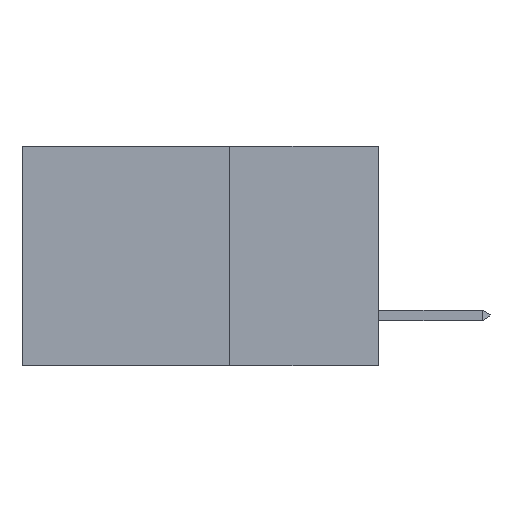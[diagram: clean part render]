
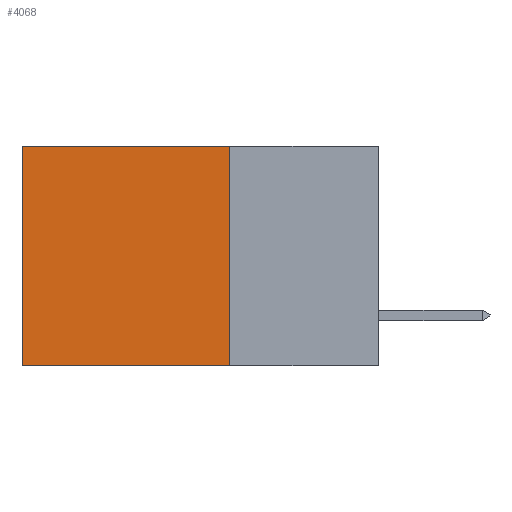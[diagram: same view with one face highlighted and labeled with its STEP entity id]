
A CAD part, left-side view. The second image highlights one B-rep face of the part: STEP entity #4068.
In plain terms, the highlighted planar face has unit normal (-1, 0, 0).
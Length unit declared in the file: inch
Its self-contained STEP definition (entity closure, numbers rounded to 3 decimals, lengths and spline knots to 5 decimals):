
#533 = DIRECTION ( 'NONE',  ( 0., 0., -1. ) ) ;
#1147 = LINE ( 'NONE', #7698, #16302 ) ;
#1148 = DIRECTION ( 'NONE',  ( 0., 0., -1. ) ) ;
#1410 = CARTESIAN_POINT ( 'NONE',  ( 0.2615, 0.25, -0.37 ) ) ;
#2628 = EDGE_LOOP ( 'NONE', ( #19874, #8429, #19953, #14181 ) ) ;
#3042 = EDGE_CURVE ( 'NONE', #7414, #20950, #13344, .T. ) ;
#4068 = ADVANCED_FACE ( 'NONE', ( #11348 ), #14703, .F. ) ;
#4478 = DIRECTION ( 'NONE',  ( 1., 0., 0. ) ) ;
#6348 = CARTESIAN_POINT ( 'NONE',  ( 0.2615, 0.25, -0.37 ) ) ;
#7414 = VERTEX_POINT ( 'NONE', #17728 ) ;
#7698 = CARTESIAN_POINT ( 'NONE',  ( 0.2615, 0.25, -0.37 ) ) ;
#7756 = VECTOR ( 'NONE', #13447, 39.37008 ) ;
#8429 = ORIENTED_EDGE ( 'NONE', *, *, #12754, .F. ) ;
#8626 = CARTESIAN_POINT ( 'NONE',  ( 0.2615, 0.6, -0.37 ) ) ;
#8818 = CARTESIAN_POINT ( 'NONE',  ( 0.2615, 0.6, 0. ) ) ;
#8958 = CARTESIAN_POINT ( 'NONE',  ( 0.2615, 0.25, -0.37 ) ) ;
#9487 = VECTOR ( 'NONE', #533, 39.37008 ) ;
#10352 = AXIS2_PLACEMENT_3D ( 'NONE', #6348, #4478, #1148 ) ;
#10924 = EDGE_CURVE ( 'NONE', #20950, #11629, #19082, .T. ) ;
#10967 = EDGE_CURVE ( 'NONE', #7414, #18882, #17422, .T. ) ;
#11257 = VECTOR ( 'NONE', #19298, 39.37008 ) ;
#11348 = FACE_OUTER_BOUND ( 'NONE', #2628, .T. ) ;
#11629 = VERTEX_POINT ( 'NONE', #21600 ) ;
#12754 = EDGE_CURVE ( 'NONE', #18882, #11629, #1147, .T. ) ;
#13344 = LINE ( 'NONE', #18709, #7756 ) ;
#13447 = DIRECTION ( 'NONE',  ( 0., 1., 0. ) ) ;
#14181 = ORIENTED_EDGE ( 'NONE', *, *, #3042, .T. ) ;
#14703 = PLANE ( 'NONE',  #10352 ) ;
#16166 = DIRECTION ( 'NONE',  ( 0., 1., 0. ) ) ;
#16302 = VECTOR ( 'NONE', #16166, 39.37008 ) ;
#17422 = LINE ( 'NONE', #8958, #11257 ) ;
#17728 = CARTESIAN_POINT ( 'NONE',  ( 0.2615, 0.25, 0. ) ) ;
#18709 = CARTESIAN_POINT ( 'NONE',  ( 0.2615, 0.25, 0. ) ) ;
#18882 = VERTEX_POINT ( 'NONE', #1410 ) ;
#19082 = LINE ( 'NONE', #8626, #9487 ) ;
#19298 = DIRECTION ( 'NONE',  ( 0., 0., -1. ) ) ;
#19874 = ORIENTED_EDGE ( 'NONE', *, *, #10924, .T. ) ;
#19953 = ORIENTED_EDGE ( 'NONE', *, *, #10967, .F. ) ;
#20950 = VERTEX_POINT ( 'NONE', #8818 ) ;
#21600 = CARTESIAN_POINT ( 'NONE',  ( 0.2615, 0.6, -0.37 ) ) ;
